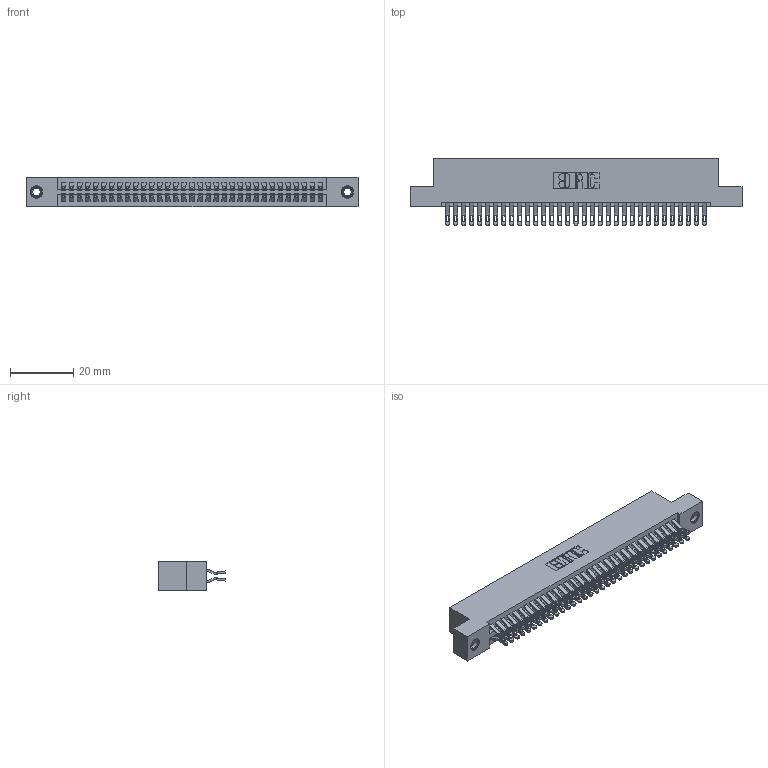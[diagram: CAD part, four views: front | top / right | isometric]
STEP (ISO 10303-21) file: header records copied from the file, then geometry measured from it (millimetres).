
FILE_DESCRIPTION (( 'STEP AP203' ), '1' );
FILE_NAME ('345-066-555-207.STEP', '2018-09-28T23:12:38', ( '' ), ( '' ), 'SwSTEP 2.0', 'SolidWorks 2016', '' );
FILE_SCHEMA (( 'CONFIG_CONTROL_DESIGN' ));
Length unit declared in the file: inch
Products named in the file (4): 345-066-555-207; 345-250-001_345-250-005-103; 345 Part_Flush Mounting Lugs - 0.156 Dia-TI; 345-292-001_555 Tail
Assembly tree (69 placements, depth 2):
  345-066-555-207
    345 Part_Flush Mounting Lugs - 0.156 Dia-TI
    345-292-001_555 Tail  x66
    345-250-001_345-250-005-103  x2
Bounding box: 105.03 x 21.13 x 9.4 mm (x, y, z)
Volume: 10297 mm3; surface area: 15740.1 mm2
Topology: 69 solids, 69 shells, 3882 faces, 12159 edges, 8098 vertices
Faces by surface type: plane 2158, cylinder 1708, cone 12, torus 4
Entity records: 28616 total; most frequent: CARTESIAN_POINT 4821, ORIENTED_EDGE 4718, DIRECTION 4257, EDGE_CURVE 2359, VECTOR 2055, LINE 2055, VERTEX_POINT 1568, AXIS2_PLACEMENT_3D 1101
